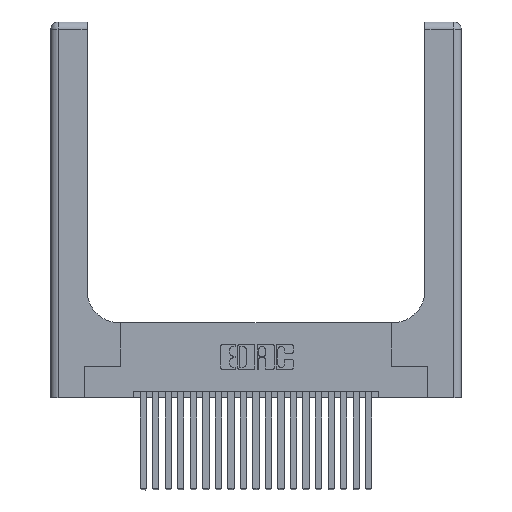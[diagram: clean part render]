
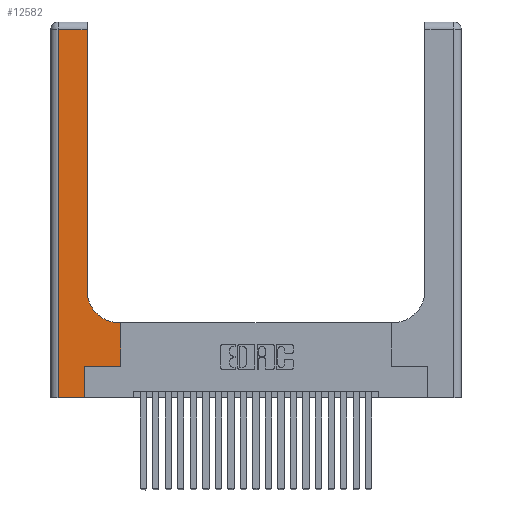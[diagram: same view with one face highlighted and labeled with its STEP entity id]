
A CAD part, top view. The second image highlights one B-rep face of the part: STEP entity #12582.
In plain terms, the highlighted planar face has unit normal (0, 0, 1).
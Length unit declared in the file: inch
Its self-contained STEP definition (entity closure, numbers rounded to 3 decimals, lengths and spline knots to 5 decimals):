
#15 = CARTESIAN_POINT ( 'NONE',  ( 0., 3., 0.37 ) ) ;
#118 = LINE ( 'NONE', #20182, #3720 ) ;
#250 = PLANE ( 'NONE',  #5059 ) ;
#1074 = VECTOR ( 'NONE', #5407, 39.37008 ) ;
#1484 = DIRECTION ( 'NONE',  ( 1., 0., 0. ) ) ;
#1641 = EDGE_CURVE ( 'NONE', #3074, #12111, #118, .T. ) ;
#1743 = CARTESIAN_POINT ( 'NONE',  ( 0.269, 0., 0.37 ) ) ;
#1932 = VERTEX_POINT ( 'NONE', #1743 ) ;
#1957 = DIRECTION ( 'NONE',  ( 0., -1., 0. ) ) ;
#2016 = DIRECTION ( 'NONE',  ( 0., 0., -1. ) ) ;
#2084 = EDGE_CURVE ( 'NONE', #4187, #3074, #13731, .T. ) ;
#2362 = EDGE_CURVE ( 'NONE', #17938, #1932, #16507, .T. ) ;
#2551 = CARTESIAN_POINT ( 'NONE',  ( 0.2915, 2.94, 0.37 ) ) ;
#2571 = ORIENTED_EDGE ( 'NONE', *, *, #5257, .T. ) ;
#2730 = EDGE_CURVE ( 'NONE', #12111, #17938, #14513, .T. ) ;
#3074 = VERTEX_POINT ( 'NONE', #2551 ) ;
#3197 = VERTEX_POINT ( 'NONE', #12009 ) ;
#3720 = VECTOR ( 'NONE', #14930, 39.37008 ) ;
#4044 = CARTESIAN_POINT ( 'NONE',  ( 0.5585, 0.6, 0.37 ) ) ;
#4186 = EDGE_CURVE ( 'NONE', #19487, #4187, #8433, .T. ) ;
#4187 = VERTEX_POINT ( 'NONE', #18524 ) ;
#4834 = DIRECTION ( 'NONE',  ( 1., 0., 0. ) ) ;
#5059 = AXIS2_PLACEMENT_3D ( 'NONE', #15, #2016, #14473 ) ;
#5257 = EDGE_CURVE ( 'NONE', #1932, #11030, #10603, .T. ) ;
#5376 = CARTESIAN_POINT ( 'NONE',  ( 0., 0., 0.37 ) ) ;
#5407 = DIRECTION ( 'NONE',  ( -1., 0., 0. ) ) ;
#5724 = VERTEX_POINT ( 'NONE', #4044 ) ;
#6317 = DIRECTION ( 'NONE',  ( 0., 1., 0. ) ) ;
#7171 = EDGE_CURVE ( 'NONE', #3197, #5724, #8853, .T. ) ;
#7298 = EDGE_CURVE ( 'NONE', #5724, #19487, #16089, .T. ) ;
#7743 = VECTOR ( 'NONE', #10849, 39.37008 ) ;
#8178 = CARTESIAN_POINT ( 'NONE',  ( 0.5415, 0.85, 0.37 ) ) ;
#8343 = ORIENTED_EDGE ( 'NONE', *, *, #1641, .T. ) ;
#8433 = CIRCLE ( 'NONE', #22648, 0.25 ) ;
#8853 = LINE ( 'NONE', #14195, #7743 ) ;
#8952 = EDGE_CURVE ( 'NONE', #11030, #3197, #9624, .T. ) ;
#9306 = ORIENTED_EDGE ( 'NONE', *, *, #2362, .T. ) ;
#9624 = LINE ( 'NONE', #16778, #21012 ) ;
#9891 = CARTESIAN_POINT ( 'NONE',  ( 0.269, 0.25, 0.37 ) ) ;
#10603 = LINE ( 'NONE', #17429, #20605 ) ;
#10849 = DIRECTION ( 'NONE',  ( 0., 1., 0. ) ) ;
#11030 = VERTEX_POINT ( 'NONE', #9891 ) ;
#12009 = CARTESIAN_POINT ( 'NONE',  ( 0.5585, 0.25, 0.37 ) ) ;
#12111 = VERTEX_POINT ( 'NONE', #14058 ) ;
#12346 = ORIENTED_EDGE ( 'NONE', *, *, #7298, .T. ) ;
#12501 = CARTESIAN_POINT ( 'NONE',  ( 0.2915, 0.6, 0.37 ) ) ;
#12582 = ADVANCED_FACE ( 'NONE', ( #19976 ), #250, .F. ) ;
#12647 = CARTESIAN_POINT ( 'NONE',  ( 0.06, 3., 0.37 ) ) ;
#13347 = DIRECTION ( 'NONE',  ( 1., 0., 0. ) ) ;
#13450 = ORIENTED_EDGE ( 'NONE', *, *, #7171, .T. ) ;
#13631 = DIRECTION ( 'NONE',  ( 0., 0., -1. ) ) ;
#13731 = LINE ( 'NONE', #20519, #21793 ) ;
#14058 = CARTESIAN_POINT ( 'NONE',  ( 0.06, 2.94, 0.37 ) ) ;
#14177 = CARTESIAN_POINT ( 'NONE',  ( 0.5415, 0.6, 0.37 ) ) ;
#14195 = CARTESIAN_POINT ( 'NONE',  ( 0.5585, 0.25, 0.37 ) ) ;
#14280 = CARTESIAN_POINT ( 'NONE',  ( 0.06, 0., 0.37 ) ) ;
#14473 = DIRECTION ( 'NONE',  ( -1., 0., 0. ) ) ;
#14513 = LINE ( 'NONE', #12647, #21461 ) ;
#14930 = DIRECTION ( 'NONE',  ( -1., 0., 0. ) ) ;
#15234 = EDGE_LOOP ( 'NONE', ( #15354, #8343, #17029, #9306, #2571, #15465, #13450, #12346, #15514 ) ) ;
#15354 = ORIENTED_EDGE ( 'NONE', *, *, #2084, .T. ) ;
#15465 = ORIENTED_EDGE ( 'NONE', *, *, #8952, .T. ) ;
#15514 = ORIENTED_EDGE ( 'NONE', *, *, #4186, .T. ) ;
#16089 = LINE ( 'NONE', #12501, #1074 ) ;
#16507 = LINE ( 'NONE', #5376, #20636 ) ;
#16778 = CARTESIAN_POINT ( 'NONE',  ( 0.269, 0.25, 0.37 ) ) ;
#17029 = ORIENTED_EDGE ( 'NONE', *, *, #2730, .T. ) ;
#17429 = CARTESIAN_POINT ( 'NONE',  ( 0.269, 0., 0.37 ) ) ;
#17938 = VERTEX_POINT ( 'NONE', #14280 ) ;
#18524 = CARTESIAN_POINT ( 'NONE',  ( 0.2915, 0.85, 0.37 ) ) ;
#19487 = VERTEX_POINT ( 'NONE', #14177 ) ;
#19976 = FACE_OUTER_BOUND ( 'NONE', #15234, .T. ) ;
#20182 = CARTESIAN_POINT ( 'NONE',  ( 0., 2.94, 0.37 ) ) ;
#20519 = CARTESIAN_POINT ( 'NONE',  ( 0.2915, 3., 0.37 ) ) ;
#20605 = VECTOR ( 'NONE', #22569, 39.37008 ) ;
#20636 = VECTOR ( 'NONE', #1484, 39.37008 ) ;
#21012 = VECTOR ( 'NONE', #13347, 39.37008 ) ;
#21461 = VECTOR ( 'NONE', #1957, 39.37008 ) ;
#21793 = VECTOR ( 'NONE', #6317, 39.37008 ) ;
#22569 = DIRECTION ( 'NONE',  ( 0., 1., 0. ) ) ;
#22648 = AXIS2_PLACEMENT_3D ( 'NONE', #8178, #13631, #4834 ) ;
